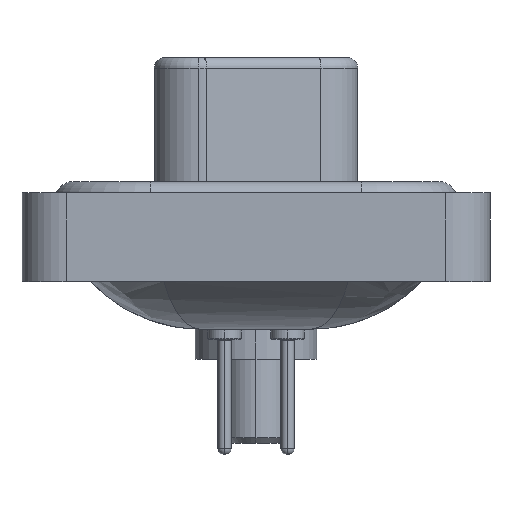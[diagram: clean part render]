
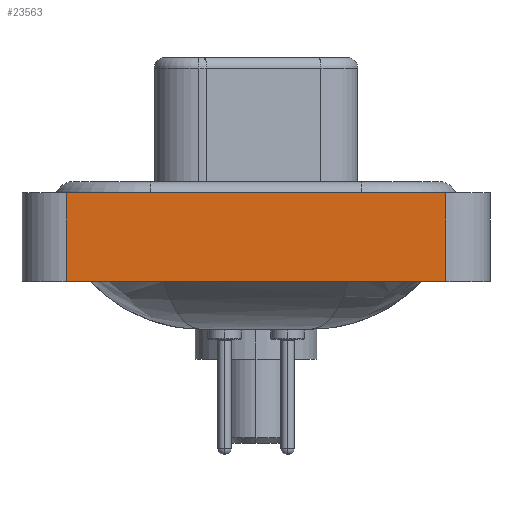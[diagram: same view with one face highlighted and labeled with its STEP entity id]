
A CAD part, left-side view. The second image highlights one B-rep face of the part: STEP entity #23563.
In plain terms, the highlighted planar face has unit normal (-1, 0, 0).
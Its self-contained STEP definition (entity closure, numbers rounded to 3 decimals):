
#157 = FACE_OUTER_BOUND ( 'NONE', #13384, .T. ) ;
#791 = CARTESIAN_POINT ( 'NONE',  ( -7.35, 8.55, -3.6 ) ) ;
#844 = CARTESIAN_POINT ( 'NONE',  ( -7.35, -8.55, -3.6 ) ) ;
#943 = LINE ( 'NONE', #17742, #11419 ) ;
#1216 = VECTOR ( 'NONE', #9166, 1000. ) ;
#2582 = CARTESIAN_POINT ( 'NONE',  ( -7.35, 8.55, -3.6 ) ) ;
#3652 = CARTESIAN_POINT ( 'NONE',  ( -7.35, 8.55, 0.4 ) ) ;
#4257 = DIRECTION ( 'NONE',  ( 0., 0., 1. ) ) ;
#4500 = VERTEX_POINT ( 'NONE', #844 ) ;
#5810 = CARTESIAN_POINT ( 'NONE',  ( -7.35, -8.55, -3.6 ) ) ;
#6263 = CARTESIAN_POINT ( 'NONE',  ( -7.35, -8.55, -3.6 ) ) ;
#6676 = VERTEX_POINT ( 'NONE', #3652 ) ;
#6935 = LINE ( 'NONE', #9296, #1216 ) ;
#7148 = VECTOR ( 'NONE', #13461, 1000. ) ;
#7461 = ORIENTED_EDGE ( 'NONE', *, *, #7479, .F. ) ;
#7479 = EDGE_CURVE ( 'NONE', #6676, #14221, #6935, .T. ) ;
#8703 = ORIENTED_EDGE ( 'NONE', *, *, #8945, .T. ) ;
#8763 = EDGE_CURVE ( 'NONE', #9024, #6676, #10204, .T. ) ;
#8945 = EDGE_CURVE ( 'NONE', #9024, #4500, #13591, .T. ) ;
#9024 = VERTEX_POINT ( 'NONE', #2582 ) ;
#9166 = DIRECTION ( 'NONE',  ( 0., -1., 0. ) ) ;
#9296 = CARTESIAN_POINT ( 'NONE',  ( -7.35, -8.55, 0.4 ) ) ;
#10204 = LINE ( 'NONE', #791, #22159 ) ;
#11419 = VECTOR ( 'NONE', #4257, 1000. ) ;
#11552 = DIRECTION ( 'NONE',  ( -1., 0., 0. ) ) ;
#11959 = AXIS2_PLACEMENT_3D ( 'NONE', #5810, #11552, #19041 ) ;
#12311 = DIRECTION ( 'NONE',  ( 0., 0., 1. ) ) ;
#13384 = EDGE_LOOP ( 'NONE', ( #22601, #7461, #20456, #8703 ) ) ;
#13461 = DIRECTION ( 'NONE',  ( 0., -1., 0. ) ) ;
#13591 = LINE ( 'NONE', #6263, #7148 ) ;
#14221 = VERTEX_POINT ( 'NONE', #20217 ) ;
#17064 = EDGE_CURVE ( 'NONE', #4500, #14221, #943, .T. ) ;
#17742 = CARTESIAN_POINT ( 'NONE',  ( -7.35, -8.55, -3.6 ) ) ;
#19041 = DIRECTION ( 'NONE',  ( 0., 0., 1. ) ) ;
#20217 = CARTESIAN_POINT ( 'NONE',  ( -7.35, -8.55, 0.4 ) ) ;
#20456 = ORIENTED_EDGE ( 'NONE', *, *, #8763, .F. ) ;
#22159 = VECTOR ( 'NONE', #12311, 1000. ) ;
#22601 = ORIENTED_EDGE ( 'NONE', *, *, #17064, .T. ) ;
#23563 = ADVANCED_FACE ( 'NONE', ( #157 ), #24371, .T. ) ;
#24371 = PLANE ( 'NONE',  #11959 ) ;
